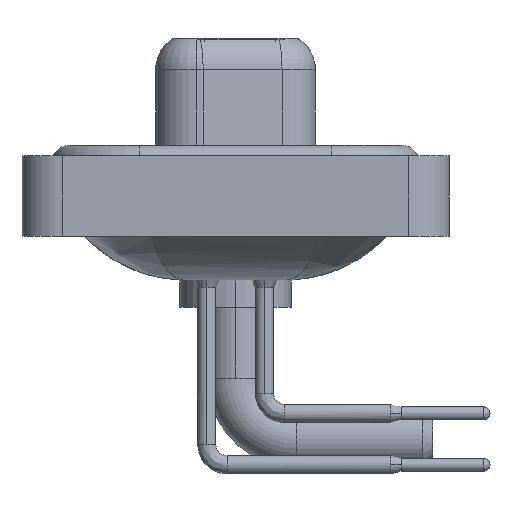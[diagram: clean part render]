
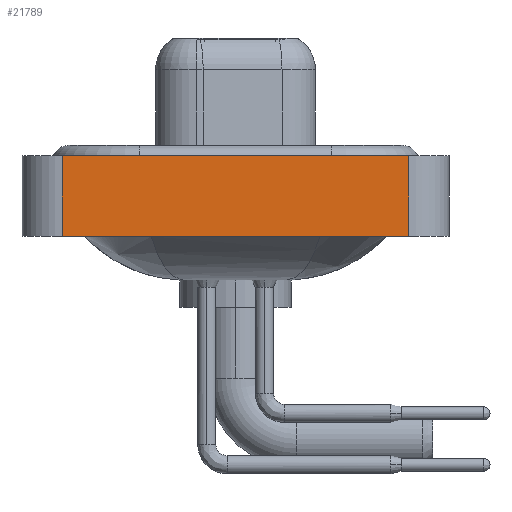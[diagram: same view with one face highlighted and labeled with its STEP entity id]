
A CAD part, left-side view. The second image highlights one B-rep face of the part: STEP entity #21789.
In plain terms, the highlighted planar face has unit normal (-1, 0, 0).
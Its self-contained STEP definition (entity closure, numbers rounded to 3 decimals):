
#275 = EDGE_CURVE ( 'NONE', #14762, #5668, #4753, .T. ) ;
#1343 = DIRECTION ( 'NONE',  ( 0., -1., 0. ) ) ;
#1461 = VERTEX_POINT ( 'NONE', #21316 ) ;
#1527 = VECTOR ( 'NONE', #7161, 1000. ) ;
#2253 = EDGE_CURVE ( 'NONE', #7207, #14762, #10662, .T. ) ;
#4753 = LINE ( 'NONE', #21959, #9589 ) ;
#4795 = VECTOR ( 'NONE', #21192, 1000. ) ;
#5668 = VERTEX_POINT ( 'NONE', #12649 ) ;
#6510 = AXIS2_PLACEMENT_3D ( 'NONE', #18568, #11477, #11579 ) ;
#7161 = DIRECTION ( 'NONE',  ( 0., 0., 1. ) ) ;
#7207 = VERTEX_POINT ( 'NONE', #18609 ) ;
#7336 = LINE ( 'NONE', #17607, #4795 ) ;
#8778 = EDGE_LOOP ( 'NONE', ( #21620, #18641, #14492, #12909 ) ) ;
#9144 = EDGE_CURVE ( 'NONE', #1461, #5668, #7336, .T. ) ;
#9589 = VECTOR ( 'NONE', #1343, 1000. ) ;
#10662 = LINE ( 'NONE', #15718, #1527 ) ;
#11477 = DIRECTION ( 'NONE',  ( -1., 0., 0. ) ) ;
#11579 = DIRECTION ( 'NONE',  ( 0., 0., 1. ) ) ;
#12147 = DIRECTION ( 'NONE',  ( 0., -1., 0. ) ) ;
#12649 = CARTESIAN_POINT ( 'NONE',  ( -7.3, -8.55, 0.4 ) ) ;
#12909 = ORIENTED_EDGE ( 'NONE', *, *, #16010, .T. ) ;
#13050 = FACE_OUTER_BOUND ( 'NONE', #8778, .T. ) ;
#13449 = VECTOR ( 'NONE', #12147, 1000. ) ;
#14492 = ORIENTED_EDGE ( 'NONE', *, *, #2253, .F. ) ;
#14762 = VERTEX_POINT ( 'NONE', #17112 ) ;
#15718 = CARTESIAN_POINT ( 'NONE',  ( -7.3, 8.55, -3.6 ) ) ;
#16010 = EDGE_CURVE ( 'NONE', #7207, #1461, #19249, .T. ) ;
#17112 = CARTESIAN_POINT ( 'NONE',  ( -7.3, 8.55, 0.4 ) ) ;
#17229 = CARTESIAN_POINT ( 'NONE',  ( -7.3, -8.55, -3.6 ) ) ;
#17607 = CARTESIAN_POINT ( 'NONE',  ( -7.3, -8.55, -3.6 ) ) ;
#18568 = CARTESIAN_POINT ( 'NONE',  ( -7.3, -8.55, -3.6 ) ) ;
#18609 = CARTESIAN_POINT ( 'NONE',  ( -7.3, 8.55, -3.6 ) ) ;
#18641 = ORIENTED_EDGE ( 'NONE', *, *, #275, .F. ) ;
#19249 = LINE ( 'NONE', #17229, #13449 ) ;
#19921 = PLANE ( 'NONE',  #6510 ) ;
#21192 = DIRECTION ( 'NONE',  ( 0., 0., 1. ) ) ;
#21316 = CARTESIAN_POINT ( 'NONE',  ( -7.3, -8.55, -3.6 ) ) ;
#21620 = ORIENTED_EDGE ( 'NONE', *, *, #9144, .T. ) ;
#21789 = ADVANCED_FACE ( 'NONE', ( #13050 ), #19921, .T. ) ;
#21959 = CARTESIAN_POINT ( 'NONE',  ( -7.3, -8.55, 0.4 ) ) ;
